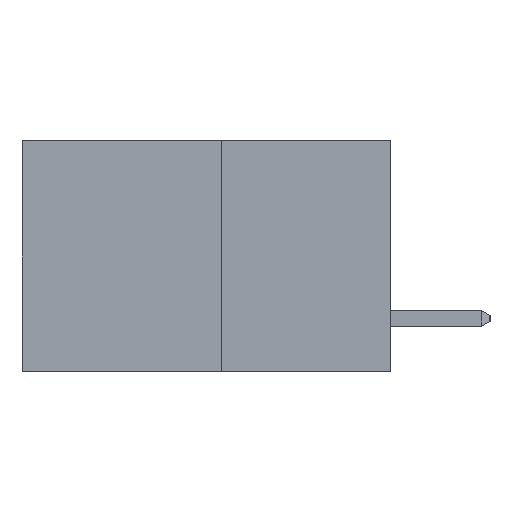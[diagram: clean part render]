
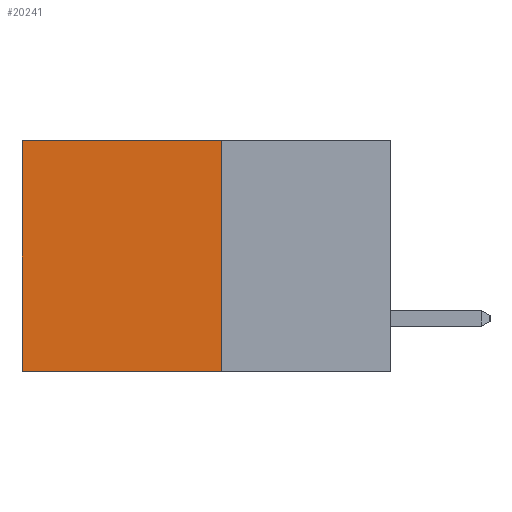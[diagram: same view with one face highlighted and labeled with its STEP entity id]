
A CAD part, left-side view. The second image highlights one B-rep face of the part: STEP entity #20241.
In plain terms, the highlighted planar face has unit normal (-1, 0, 0).
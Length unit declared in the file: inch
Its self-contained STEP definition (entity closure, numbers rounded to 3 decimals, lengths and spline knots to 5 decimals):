
#112 = VECTOR ( 'NONE', #14258, 39.37008 ) ;
#1116 = DIRECTION ( 'NONE',  ( 1., 0., 0. ) ) ;
#3096 = ORIENTED_EDGE ( 'NONE', *, *, #28114, .T. ) ;
#6401 = LINE ( 'NONE', #7143, #112 ) ;
#6458 = CARTESIAN_POINT ( 'NONE',  ( 0.277, 0.27, 0. ) ) ;
#7143 = CARTESIAN_POINT ( 'NONE',  ( 0.277, 0.59, -0.37 ) ) ;
#7580 = VERTEX_POINT ( 'NONE', #9049 ) ;
#7898 = ORIENTED_EDGE ( 'NONE', *, *, #8259, .F. ) ;
#8259 = EDGE_CURVE ( 'NONE', #15354, #15228, #18809, .T. ) ;
#8700 = VECTOR ( 'NONE', #25092, 39.37008 ) ;
#9049 = CARTESIAN_POINT ( 'NONE',  ( 0.277, 0.59, 0. ) ) ;
#9584 = ORIENTED_EDGE ( 'NONE', *, *, #14228, .T. ) ;
#9854 = EDGE_CURVE ( 'NONE', #15228, #12984, #14632, .T. ) ;
#12531 = VECTOR ( 'NONE', #28017, 39.37008 ) ;
#12984 = VERTEX_POINT ( 'NONE', #14111 ) ;
#14111 = CARTESIAN_POINT ( 'NONE',  ( 0.277, 0.59, -0.37 ) ) ;
#14228 = EDGE_CURVE ( 'NONE', #7580, #12984, #6401, .T. ) ;
#14258 = DIRECTION ( 'NONE',  ( 0., 0., -1. ) ) ;
#14632 = LINE ( 'NONE', #24325, #26478 ) ;
#14993 = FACE_OUTER_BOUND ( 'NONE', #18217, .T. ) ;
#15228 = VERTEX_POINT ( 'NONE', #29593 ) ;
#15255 = PLANE ( 'NONE',  #21741 ) ;
#15354 = VERTEX_POINT ( 'NONE', #6458 ) ;
#15569 = CARTESIAN_POINT ( 'NONE',  ( 0.277, 0.27, 0. ) ) ;
#16131 = CARTESIAN_POINT ( 'NONE',  ( 0.277, 0.27, -0.37 ) ) ;
#17637 = DIRECTION ( 'NONE',  ( 0., 0., -1. ) ) ;
#18217 = EDGE_LOOP ( 'NONE', ( #9584, #18372, #7898, #3096 ) ) ;
#18372 = ORIENTED_EDGE ( 'NONE', *, *, #9854, .F. ) ;
#18809 = LINE ( 'NONE', #16131, #12531 ) ;
#20241 = ADVANCED_FACE ( 'NONE', ( #14993 ), #15255, .F. ) ;
#21741 = AXIS2_PLACEMENT_3D ( 'NONE', #24689, #1116, #17637 ) ;
#24325 = CARTESIAN_POINT ( 'NONE',  ( 0.277, 0.27, -0.37 ) ) ;
#24689 = CARTESIAN_POINT ( 'NONE',  ( 0.277, 0.27, -0.37 ) ) ;
#25092 = DIRECTION ( 'NONE',  ( 0., 1., 0. ) ) ;
#26478 = VECTOR ( 'NONE', #29075, 39.37008 ) ;
#27548 = LINE ( 'NONE', #15569, #8700 ) ;
#28017 = DIRECTION ( 'NONE',  ( 0., 0., -1. ) ) ;
#28114 = EDGE_CURVE ( 'NONE', #15354, #7580, #27548, .T. ) ;
#29075 = DIRECTION ( 'NONE',  ( 0., 1., 0. ) ) ;
#29593 = CARTESIAN_POINT ( 'NONE',  ( 0.277, 0.27, -0.37 ) ) ;
